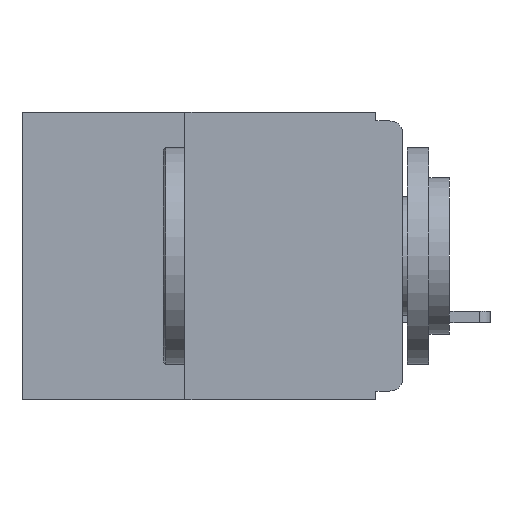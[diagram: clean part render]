
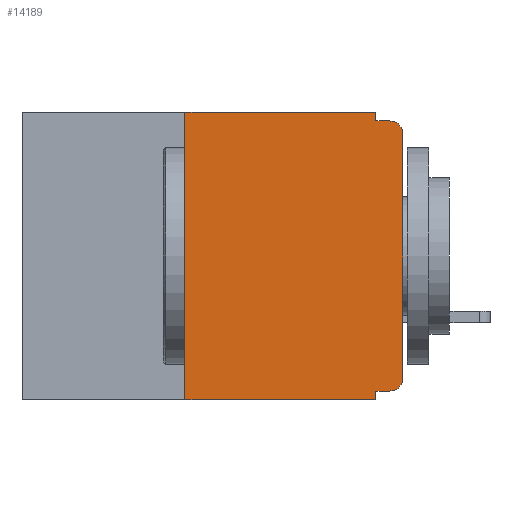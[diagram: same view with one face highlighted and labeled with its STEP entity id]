
A CAD part, left-side view. The second image highlights one B-rep face of the part: STEP entity #14189.
In plain terms, the highlighted planar face has unit normal (-1, 0, 0).
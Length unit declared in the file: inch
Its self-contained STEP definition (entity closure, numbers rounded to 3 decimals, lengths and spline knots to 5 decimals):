
#187 = ORIENTED_EDGE ( 'NONE', *, *, #13827, .F. ) ;
#398 = VERTEX_POINT ( 'NONE', #7251 ) ;
#565 = ORIENTED_EDGE ( 'NONE', *, *, #11014, .F. ) ;
#923 = DIRECTION ( 'NONE',  ( 0., 1., 0. ) ) ;
#969 = CARTESIAN_POINT ( 'NONE',  ( 0., 0., -0.32 ) ) ;
#1282 = EDGE_LOOP ( 'NONE', ( #18839, #7652, #565, #20598, #3409, #3072, #10601, #187, #12110, #18728 ) ) ;
#1471 = VERTEX_POINT ( 'NONE', #20385 ) ;
#2016 = VECTOR ( 'NONE', #923, 39.37008 ) ;
#2267 = LINE ( 'NONE', #11629, #14819 ) ;
#3072 = ORIENTED_EDGE ( 'NONE', *, *, #18189, .F. ) ;
#3288 = LINE ( 'NONE', #20632, #11480 ) ;
#3409 = ORIENTED_EDGE ( 'NONE', *, *, #13884, .F. ) ;
#3417 = VERTEX_POINT ( 'NONE', #17564 ) ;
#3946 = FACE_OUTER_BOUND ( 'NONE', #1282, .T. ) ;
#4285 = DIRECTION ( 'NONE',  ( 0., -1., 0. ) ) ;
#4715 = VECTOR ( 'NONE', #17897, 39.37008 ) ;
#4903 = CARTESIAN_POINT ( 'NONE',  ( 0., 0.437, -0.33 ) ) ;
#5804 = VERTEX_POINT ( 'NONE', #8265 ) ;
#6272 = EDGE_CURVE ( 'NONE', #9441, #398, #10763, .T. ) ;
#6444 = CARTESIAN_POINT ( 'NONE',  ( 0., 0.015, -0.305 ) ) ;
#6855 = VERTEX_POINT ( 'NONE', #12587 ) ;
#7099 = CARTESIAN_POINT ( 'NONE',  ( 0., 0.031, 0. ) ) ;
#7251 = CARTESIAN_POINT ( 'NONE',  ( 0., 0.031, -0.32 ) ) ;
#7308 = AXIS2_PLACEMENT_3D ( 'NONE', #14995, #19823, #10157 ) ;
#7319 = DIRECTION ( 'NONE',  ( 0., 0., 1. ) ) ;
#7451 = EDGE_CURVE ( 'NONE', #17957, #6855, #12407, .T. ) ;
#7556 = CARTESIAN_POINT ( 'NONE',  ( 0., 0.437, 0. ) ) ;
#7652 = ORIENTED_EDGE ( 'NONE', *, *, #11409, .T. ) ;
#7732 = DIRECTION ( 'NONE',  ( -1., 0., 0. ) ) ;
#7806 = CARTESIAN_POINT ( 'NONE',  ( 0., 0., -0.025 ) ) ;
#8016 = VECTOR ( 'NONE', #7319, 39.37008 ) ;
#8097 = DIRECTION ( 'NONE',  ( 0., 0., -1. ) ) ;
#8265 = CARTESIAN_POINT ( 'NONE',  ( 0., 0., -0.305 ) ) ;
#9016 = CARTESIAN_POINT ( 'NONE',  ( 0., 0.031, -0.33 ) ) ;
#9441 = VERTEX_POINT ( 'NONE', #16491 ) ;
#9591 = VECTOR ( 'NONE', #18691, 39.37008 ) ;
#9995 = DIRECTION ( 'NONE',  ( 0., -1., 0. ) ) ;
#10157 = DIRECTION ( 'NONE',  ( 0., 0., -1. ) ) ;
#10601 = ORIENTED_EDGE ( 'NONE', *, *, #7451, .T. ) ;
#10620 = CARTESIAN_POINT ( 'NONE',  ( 0., 0.015, -0.01 ) ) ;
#10763 = LINE ( 'NONE', #969, #2016 ) ;
#11014 = EDGE_CURVE ( 'NONE', #19890, #15700, #2267, .T. ) ;
#11165 = EDGE_CURVE ( 'NONE', #3417, #19890, #20839, .T. ) ;
#11409 = EDGE_CURVE ( 'NONE', #17601, #15700, #16287, .T. ) ;
#11480 = VECTOR ( 'NONE', #15781, 39.37008 ) ;
#11629 = CARTESIAN_POINT ( 'NONE',  ( 0., 0., -0.01 ) ) ;
#11712 = PLANE ( 'NONE',  #7308 ) ;
#11893 = VECTOR ( 'NONE', #4285, 39.37008 ) ;
#11979 = DIRECTION ( 'NONE',  ( 0., 0., -1. ) ) ;
#12110 = ORIENTED_EDGE ( 'NONE', *, *, #6272, .F. ) ;
#12407 = LINE ( 'NONE', #4903, #4715 ) ;
#12587 = CARTESIAN_POINT ( 'NONE',  ( 0., 0.031, -0.33 ) ) ;
#12787 = VECTOR ( 'NONE', #11979, 39.37008 ) ;
#13608 = CARTESIAN_POINT ( 'NONE',  ( 0., 0.25, -0.33 ) ) ;
#13827 = EDGE_CURVE ( 'NONE', #398, #6855, #14443, .T. ) ;
#13884 = EDGE_CURVE ( 'NONE', #1471, #3417, #20982, .T. ) ;
#14189 = ADVANCED_FACE ( 'NONE', ( #3946 ), #11712, .F. ) ;
#14345 = EDGE_CURVE ( 'NONE', #5804, #17601, #20461, .T. ) ;
#14443 = LINE ( 'NONE', #9016, #9591 ) ;
#14819 = VECTOR ( 'NONE', #9995, 39.37008 ) ;
#14995 = CARTESIAN_POINT ( 'NONE',  ( 0., 0.437, 0. ) ) ;
#15432 = CARTESIAN_POINT ( 'NONE',  ( 0., 0.031, -0.01 ) ) ;
#15673 = AXIS2_PLACEMENT_3D ( 'NONE', #6444, #17816, #8097 ) ;
#15700 = VERTEX_POINT ( 'NONE', #10620 ) ;
#15781 = DIRECTION ( 'NONE',  ( 0., 0., 1. ) ) ;
#15875 = AXIS2_PLACEMENT_3D ( 'NONE', #17461, #7732, #19075 ) ;
#16287 = CIRCLE ( 'NONE', #15875, 0.015 ) ;
#16491 = CARTESIAN_POINT ( 'NONE',  ( 0., 0.015, -0.32 ) ) ;
#17461 = CARTESIAN_POINT ( 'NONE',  ( 0., 0.015, -0.025 ) ) ;
#17564 = CARTESIAN_POINT ( 'NONE',  ( 0., 0.031, 0. ) ) ;
#17601 = VERTEX_POINT ( 'NONE', #7806 ) ;
#17816 = DIRECTION ( 'NONE',  ( -1., 0., 0. ) ) ;
#17897 = DIRECTION ( 'NONE',  ( 0., -1., 0. ) ) ;
#17957 = VERTEX_POINT ( 'NONE', #13608 ) ;
#18189 = EDGE_CURVE ( 'NONE', #17957, #1471, #3288, .T. ) ;
#18668 = CARTESIAN_POINT ( 'NONE',  ( 0., 0., 0. ) ) ;
#18691 = DIRECTION ( 'NONE',  ( 0., 0., -1. ) ) ;
#18728 = ORIENTED_EDGE ( 'NONE', *, *, #20766, .T. ) ;
#18839 = ORIENTED_EDGE ( 'NONE', *, *, #14345, .T. ) ;
#19075 = DIRECTION ( 'NONE',  ( 0., 0., -1. ) ) ;
#19823 = DIRECTION ( 'NONE',  ( 1., 0., 0. ) ) ;
#19890 = VERTEX_POINT ( 'NONE', #15432 ) ;
#20029 = CIRCLE ( 'NONE', #15673, 0.015 ) ;
#20385 = CARTESIAN_POINT ( 'NONE',  ( 0., 0.25, 0. ) ) ;
#20461 = LINE ( 'NONE', #18668, #8016 ) ;
#20598 = ORIENTED_EDGE ( 'NONE', *, *, #11165, .F. ) ;
#20632 = CARTESIAN_POINT ( 'NONE',  ( 0., 0.25, -0.33 ) ) ;
#20766 = EDGE_CURVE ( 'NONE', #9441, #5804, #20029, .T. ) ;
#20839 = LINE ( 'NONE', #7099, #12787 ) ;
#20982 = LINE ( 'NONE', #7556, #11893 ) ;
